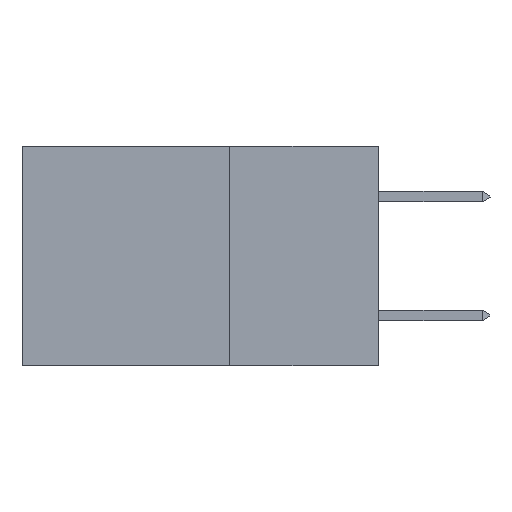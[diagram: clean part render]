
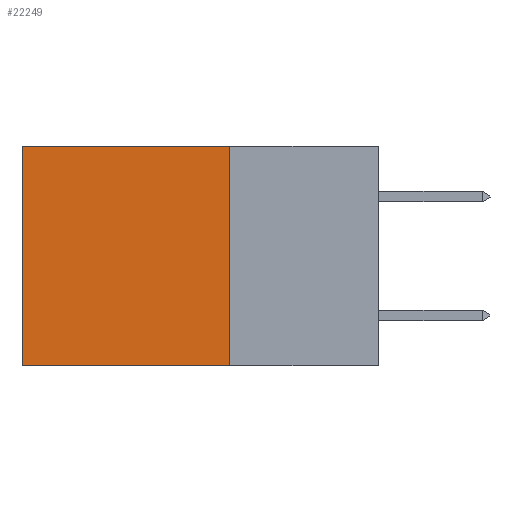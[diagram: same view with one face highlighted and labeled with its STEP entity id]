
A CAD part, left-side view. The second image highlights one B-rep face of the part: STEP entity #22249.
In plain terms, the highlighted planar face has unit normal (-1, 0, 0).
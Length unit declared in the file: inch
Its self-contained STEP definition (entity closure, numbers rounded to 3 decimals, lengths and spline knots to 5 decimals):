
#46 = DIRECTION ( 'NONE',  ( 0., 0., -1. ) ) ;
#451 = DIRECTION ( 'NONE',  ( 0., 1., 0. ) ) ;
#529 = LINE ( 'NONE', #7905, #20202 ) ;
#2680 = ORIENTED_EDGE ( 'NONE', *, *, #11286, .T. ) ;
#2683 = LINE ( 'NONE', #4740, #6345 ) ;
#3242 = VECTOR ( 'NONE', #4499, 39.37008 ) ;
#4499 = DIRECTION ( 'NONE',  ( 0., 0., -1. ) ) ;
#4740 = CARTESIAN_POINT ( 'NONE',  ( 0.298, 0.6, 0. ) ) ;
#4822 = CARTESIAN_POINT ( 'NONE',  ( 0.298, 0.6, 0. ) ) ;
#5265 = EDGE_LOOP ( 'NONE', ( #2680, #15451, #29457, #22194 ) ) ;
#6345 = VECTOR ( 'NONE', #46, 39.37008 ) ;
#7509 = DIRECTION ( 'NONE',  ( 0., 1., 0. ) ) ;
#7905 = CARTESIAN_POINT ( 'NONE',  ( 0.298, 0.25, 0. ) ) ;
#8645 = VERTEX_POINT ( 'NONE', #27730 ) ;
#11286 = EDGE_CURVE ( 'NONE', #13044, #8645, #2683, .T. ) ;
#11472 = FACE_OUTER_BOUND ( 'NONE', #5265, .T. ) ;
#13044 = VERTEX_POINT ( 'NONE', #4822 ) ;
#14375 = LINE ( 'NONE', #25844, #3242 ) ;
#15451 = ORIENTED_EDGE ( 'NONE', *, *, #22794, .F. ) ;
#18884 = DIRECTION ( 'NONE',  ( 1., 0., 0. ) ) ;
#19634 = VECTOR ( 'NONE', #7509, 39.37008 ) ;
#19710 = EDGE_CURVE ( 'NONE', #21893, #13044, #529, .T. ) ;
#20202 = VECTOR ( 'NONE', #451, 39.37008 ) ;
#21030 = AXIS2_PLACEMENT_3D ( 'NONE', #29071, #18884, #30465 ) ;
#21893 = VERTEX_POINT ( 'NONE', #23721 ) ;
#22194 = ORIENTED_EDGE ( 'NONE', *, *, #19710, .T. ) ;
#22249 = ADVANCED_FACE ( 'NONE', ( #11472 ), #22282, .F. ) ;
#22282 = PLANE ( 'NONE',  #21030 ) ;
#22794 = EDGE_CURVE ( 'NONE', #29694, #8645, #24109, .T. ) ;
#23721 = CARTESIAN_POINT ( 'NONE',  ( 0.298, 0.25, 0. ) ) ;
#23870 = EDGE_CURVE ( 'NONE', #21893, #29694, #14375, .T. ) ;
#24109 = LINE ( 'NONE', #24214, #19634 ) ;
#24214 = CARTESIAN_POINT ( 'NONE',  ( 0.298, 0.25, -0.37 ) ) ;
#25844 = CARTESIAN_POINT ( 'NONE',  ( 0.298, 0.25, 0. ) ) ;
#27730 = CARTESIAN_POINT ( 'NONE',  ( 0.298, 0.6, -0.37 ) ) ;
#29071 = CARTESIAN_POINT ( 'NONE',  ( 0.298, 0.25, 0. ) ) ;
#29457 = ORIENTED_EDGE ( 'NONE', *, *, #23870, .F. ) ;
#29694 = VERTEX_POINT ( 'NONE', #29710 ) ;
#29710 = CARTESIAN_POINT ( 'NONE',  ( 0.298, 0.25, -0.37 ) ) ;
#30465 = DIRECTION ( 'NONE',  ( 0., 0., -1. ) ) ;
